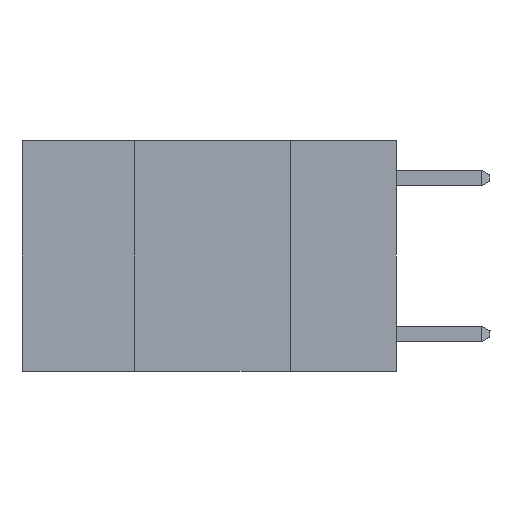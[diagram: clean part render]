
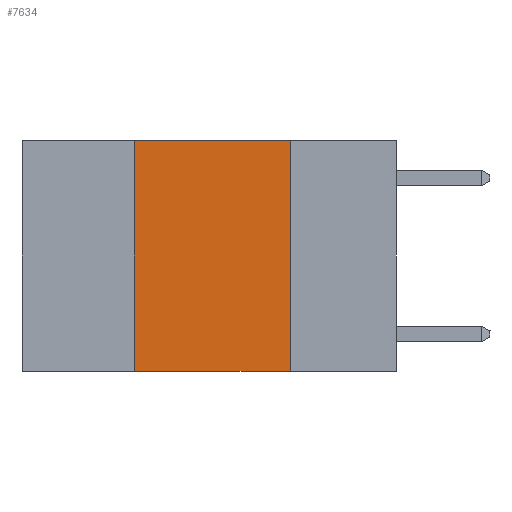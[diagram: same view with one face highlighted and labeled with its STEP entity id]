
A CAD part, left-side view. The second image highlights one B-rep face of the part: STEP entity #7634.
In plain terms, the highlighted planar face has unit normal (-1, 0, 0).
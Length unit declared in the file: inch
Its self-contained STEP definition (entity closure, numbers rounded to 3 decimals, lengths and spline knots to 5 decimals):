
#1653 = VECTOR ( 'NONE', #14384, 39.37008 ) ;
#2051 = DIRECTION ( 'NONE',  ( 0., 0., 1. ) ) ;
#2496 = DIRECTION ( 'NONE',  ( 1., 0., 0. ) ) ;
#4378 = EDGE_CURVE ( 'NONE', #10473, #15798, #10680, .T. ) ;
#4939 = EDGE_LOOP ( 'NONE', ( #20292, #24039, #18677, #6656 ) ) ;
#6623 = EDGE_CURVE ( 'NONE', #10473, #15517, #24116, .T. ) ;
#6656 = ORIENTED_EDGE ( 'NONE', *, *, #4378, .T. ) ;
#7060 = CARTESIAN_POINT ( 'NONE',  ( 0., 0.6, 0. ) ) ;
#7634 = ADVANCED_FACE ( 'NONE', ( #23456 ), #12987, .F. ) ;
#9610 = CARTESIAN_POINT ( 'NONE',  ( 0., 0.42, -0.37 ) ) ;
#10420 = DIRECTION ( 'NONE',  ( 0., -1., 0. ) ) ;
#10473 = VERTEX_POINT ( 'NONE', #9610 ) ;
#10680 = LINE ( 'NONE', #14301, #15888 ) ;
#12723 = DIRECTION ( 'NONE',  ( 0., 0., -1. ) ) ;
#12940 = VECTOR ( 'NONE', #2051, 39.37008 ) ;
#12987 = PLANE ( 'NONE',  #14248 ) ;
#13137 = CARTESIAN_POINT ( 'NONE',  ( 0., 0.17, 0. ) ) ;
#14248 = AXIS2_PLACEMENT_3D ( 'NONE', #7060, #2496, #12723 ) ;
#14301 = CARTESIAN_POINT ( 'NONE',  ( 0., 0.6, -0.37 ) ) ;
#14384 = DIRECTION ( 'NONE',  ( 0., -1., 0. ) ) ;
#15011 = VECTOR ( 'NONE', #22949, 39.37008 ) ;
#15517 = VERTEX_POINT ( 'NONE', #25823 ) ;
#15798 = VERTEX_POINT ( 'NONE', #19059 ) ;
#15888 = VECTOR ( 'NONE', #10420, 39.37008 ) ;
#16357 = EDGE_CURVE ( 'NONE', #23911, #15798, #25237, .T. ) ;
#17042 = EDGE_CURVE ( 'NONE', #15517, #23911, #18521, .T. ) ;
#18521 = LINE ( 'NONE', #24864, #1653 ) ;
#18677 = ORIENTED_EDGE ( 'NONE', *, *, #6623, .F. ) ;
#19059 = CARTESIAN_POINT ( 'NONE',  ( 0., 0.17, -0.37 ) ) ;
#20292 = ORIENTED_EDGE ( 'NONE', *, *, #16357, .F. ) ;
#20431 = CARTESIAN_POINT ( 'NONE',  ( 0., 0.42, 0. ) ) ;
#22949 = DIRECTION ( 'NONE',  ( 0., 0., -1. ) ) ;
#23276 = CARTESIAN_POINT ( 'NONE',  ( 0., 0.17, 0. ) ) ;
#23456 = FACE_OUTER_BOUND ( 'NONE', #4939, .T. ) ;
#23911 = VERTEX_POINT ( 'NONE', #23276 ) ;
#24039 = ORIENTED_EDGE ( 'NONE', *, *, #17042, .F. ) ;
#24116 = LINE ( 'NONE', #20431, #12940 ) ;
#24864 = CARTESIAN_POINT ( 'NONE',  ( 0., 0.6, 0. ) ) ;
#25237 = LINE ( 'NONE', #13137, #15011 ) ;
#25823 = CARTESIAN_POINT ( 'NONE',  ( 0., 0.42, 0. ) ) ;
